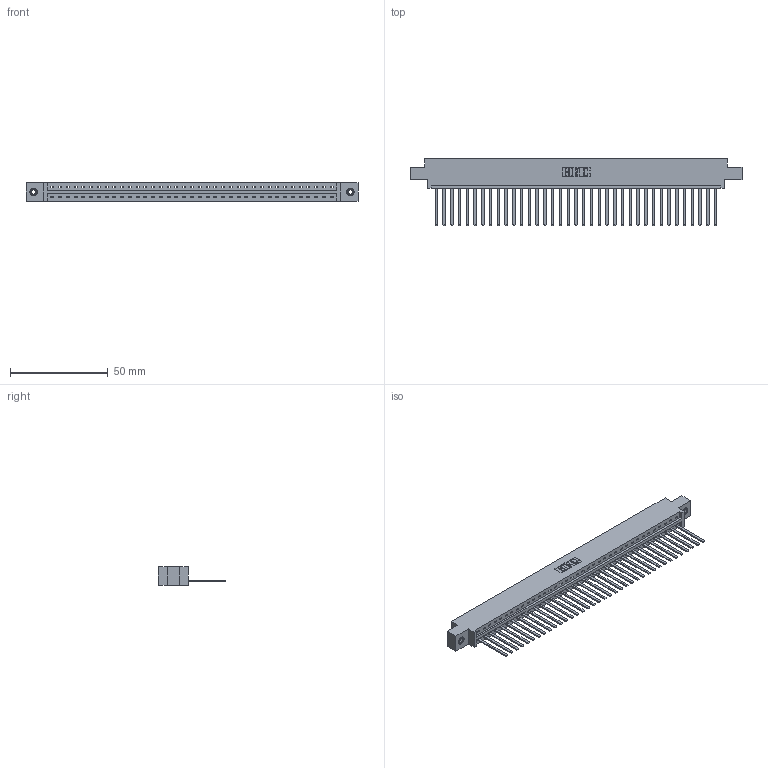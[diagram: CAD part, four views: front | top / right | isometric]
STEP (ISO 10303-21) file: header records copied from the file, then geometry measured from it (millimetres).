
FILE_DESCRIPTION (( 'STEP AP203' ), '1' );
FILE_NAME ('337-037-544-608.STEP', '2019-10-01T16:03:19', ( '' ), ( '' ), 'SwSTEP 2.0', 'SolidWorks 2016', '' );
FILE_SCHEMA (( 'CONFIG_CONTROL_DESIGN' ));
Length unit declared in the file: inch
Products named in the file (4): 337 Part_0.170 Offset - 0.156 Dia-TI; 337-037-544-608; 345-250-001_345-250-003-102; 345-292-001_345-293-144
Assembly tree (40 placements, depth 2):
  337-037-544-608
    337 Part_0.170 Offset - 0.156 Dia-TI
    345-292-001_345-293-144  x37
    345-250-001_345-250-003-102  x2
Bounding box: 169.62 x 34.3 x 9.4 mm (x, y, z)
Volume: 17871.2 mm3; surface area: 19975.2 mm2
Topology: 40 solids, 40 shells, 2250 faces, 6749 edges, 4442 vertices
Faces by surface type: plane 1660, cylinder 574, cone 12, torus 4
Entity records: 29284 total; most frequent: CARTESIAN_POINT 5080, ORIENTED_EDGE 5046, DIRECTION 4315, EDGE_CURVE 2523, VECTOR 2379, LINE 2379, VERTEX_POINT 1676, AXIS2_PLACEMENT_3D 968
